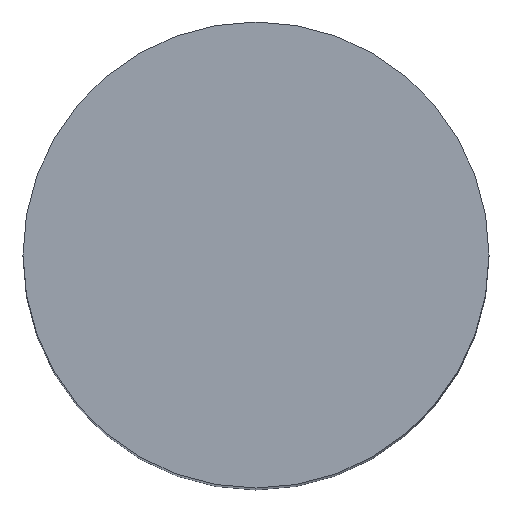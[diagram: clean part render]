
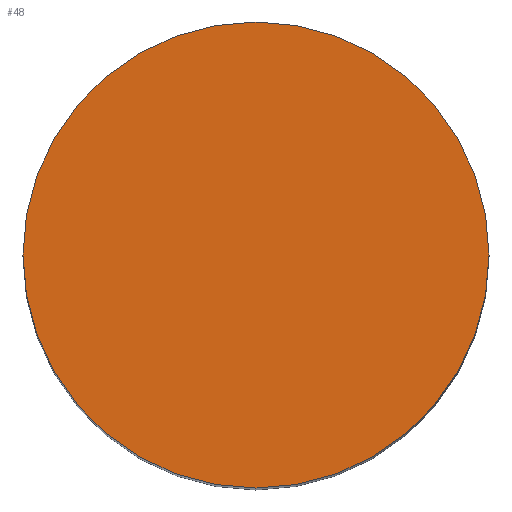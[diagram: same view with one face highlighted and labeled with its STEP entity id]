
A CAD part, top view. The second image highlights one B-rep face of the part: STEP entity #48.
In plain terms, the highlighted planar face has unit normal (0, 0, 1).
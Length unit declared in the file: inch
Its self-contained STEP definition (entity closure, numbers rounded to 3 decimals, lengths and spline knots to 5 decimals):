
#1 = CARTESIAN_POINT ( 'NONE',  ( 0., 0., 0.57087 ) ) ;
#4 = ORIENTED_EDGE ( 'NONE', *, *, #125, .T. ) ;
#6 = CIRCLE ( 'NONE', #145, 0.11811 ) ;
#8 = VERTEX_POINT ( 'NONE', #74 ) ;
#18 = FACE_OUTER_BOUND ( 'NONE', #58, .T. ) ;
#19 = DIRECTION ( 'NONE',  ( 1., 0., 0. ) ) ;
#32 = CARTESIAN_POINT ( 'NONE',  ( -0.11811, 0., 0.57087 ) ) ;
#37 = PLANE ( 'NONE',  #71 ) ;
#38 = CIRCLE ( 'NONE', #133, 0.11811 ) ;
#48 = ADVANCED_FACE ( 'NONE', ( #18 ), #37, .T. ) ;
#53 = CARTESIAN_POINT ( 'NONE',  ( 0., 0., 0.57087 ) ) ;
#58 = EDGE_LOOP ( 'NONE', ( #76, #4 ) ) ;
#63 = DIRECTION ( 'NONE',  ( 1., 0., 0. ) ) ;
#71 = AXIS2_PLACEMENT_3D ( 'NONE', #83, #99, #91 ) ;
#74 = CARTESIAN_POINT ( 'NONE',  ( 0.11811, 0., 0.57087 ) ) ;
#76 = ORIENTED_EDGE ( 'NONE', *, *, #135, .T. ) ;
#83 = CARTESIAN_POINT ( 'NONE',  ( 0., 0., 0.57087 ) ) ;
#87 = DIRECTION ( 'NONE',  ( 0., 0., 1. ) ) ;
#91 = DIRECTION ( 'NONE',  ( 1., 0., 0. ) ) ;
#99 = DIRECTION ( 'NONE',  ( 0., 0., 1. ) ) ;
#102 = VERTEX_POINT ( 'NONE', #32 ) ;
#120 = DIRECTION ( 'NONE',  ( 0., 0., 1. ) ) ;
#125 = EDGE_CURVE ( 'NONE', #8, #102, #38, .T. ) ;
#133 = AXIS2_PLACEMENT_3D ( 'NONE', #53, #120, #63 ) ;
#135 = EDGE_CURVE ( 'NONE', #102, #8, #6, .T. ) ;
#145 = AXIS2_PLACEMENT_3D ( 'NONE', #1, #87, #19 ) ;
